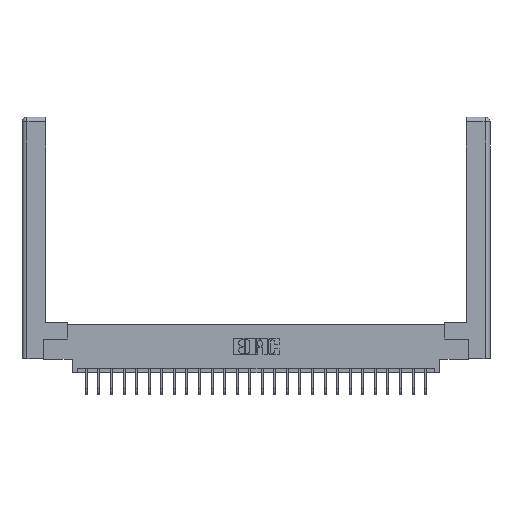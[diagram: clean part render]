
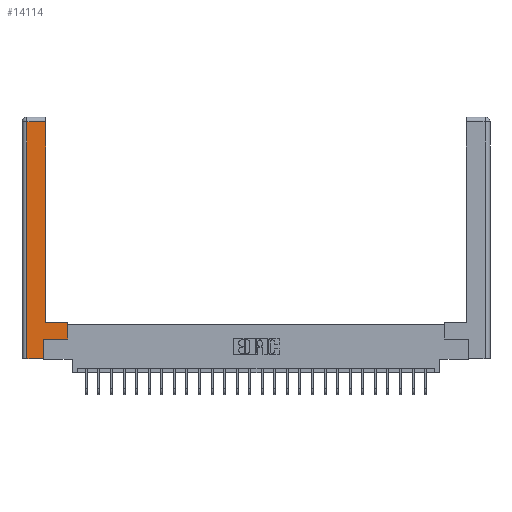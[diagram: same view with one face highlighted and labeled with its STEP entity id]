
A CAD part, top view. The second image highlights one B-rep face of the part: STEP entity #14114.
In plain terms, the highlighted planar face has unit normal (0, 0, 1).
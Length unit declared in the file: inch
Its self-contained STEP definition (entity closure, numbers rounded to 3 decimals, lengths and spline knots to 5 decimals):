
#35 = ORIENTED_EDGE ( 'NONE', *, *, #8858, .T. ) ;
#504 = EDGE_CURVE ( 'NONE', #5741, #15516, #4902, .T. ) ;
#1690 = LINE ( 'NONE', #20446, #19016 ) ;
#2625 = CARTESIAN_POINT ( 'NONE',  ( 0.565, 0.245, 0. ) ) ;
#2643 = CARTESIAN_POINT ( 'NONE',  ( 0.565, 0.45, 0. ) ) ;
#2714 = ORIENTED_EDGE ( 'NONE', *, *, #23571, .T. ) ;
#3656 = VERTEX_POINT ( 'NONE', #13217 ) ;
#4498 = ORIENTED_EDGE ( 'NONE', *, *, #504, .T. ) ;
#4645 = ORIENTED_EDGE ( 'NONE', *, *, #26272, .T. ) ;
#4902 = LINE ( 'NONE', #16597, #22898 ) ;
#5548 = DIRECTION ( 'NONE',  ( 1., 0., 0. ) ) ;
#5676 = DIRECTION ( 'NONE',  ( 0., 1., 0. ) ) ;
#5741 = VERTEX_POINT ( 'NONE', #2643 ) ;
#5812 = LINE ( 'NONE', #17185, #20409 ) ;
#6780 = CARTESIAN_POINT ( 'NONE',  ( 0.0615, 2.94, 0. ) ) ;
#6883 = VERTEX_POINT ( 'NONE', #10558 ) ;
#7050 = CARTESIAN_POINT ( 'NONE',  ( 0.265, 0.245, 0. ) ) ;
#8350 = VERTEX_POINT ( 'NONE', #18207 ) ;
#8858 = EDGE_CURVE ( 'NONE', #15516, #6883, #27271, .T. ) ;
#8948 = LINE ( 'NONE', #13601, #22228 ) ;
#9142 = ORIENTED_EDGE ( 'NONE', *, *, #23802, .T. ) ;
#9517 = CARTESIAN_POINT ( 'NONE',  ( 0.0615, 2.94, 0. ) ) ;
#10075 = DIRECTION ( 'NONE',  ( -1., 0., 0. ) ) ;
#10157 = DIRECTION ( 'NONE',  ( -1., 0., 0. ) ) ;
#10325 = CARTESIAN_POINT ( 'NONE',  ( 0.295, 3., 0. ) ) ;
#10416 = VECTOR ( 'NONE', #13216, 39.37008 ) ;
#10558 = CARTESIAN_POINT ( 'NONE',  ( 0.295, 2.94, 0. ) ) ;
#11442 = DIRECTION ( 'NONE',  ( 1., 0., 0. ) ) ;
#13006 = DIRECTION ( 'NONE',  ( 0., -1., 0. ) ) ;
#13217 = CARTESIAN_POINT ( 'NONE',  ( 0.265, 0., 0. ) ) ;
#13216 = DIRECTION ( 'NONE',  ( 0., 1., 0. ) ) ;
#13601 = CARTESIAN_POINT ( 'NONE',  ( 0.265, 0., 0. ) ) ;
#14114 = ADVANCED_FACE ( 'NONE', ( #24796 ), #27382, .F. ) ;
#14404 = DIRECTION ( 'NONE',  ( 0., 0., -1. ) ) ;
#14780 = CARTESIAN_POINT ( 'NONE',  ( 0.265, 0.245, 0. ) ) ;
#15516 = VERTEX_POINT ( 'NONE', #20172 ) ;
#16261 = ORIENTED_EDGE ( 'NONE', *, *, #25699, .T. ) ;
#16597 = CARTESIAN_POINT ( 'NONE',  ( 0.295, 0.45, 0. ) ) ;
#16770 = VECTOR ( 'NONE', #21987, 39.37008 ) ;
#17185 = CARTESIAN_POINT ( 'NONE',  ( 0.0615, 0., 0. ) ) ;
#17998 = LINE ( 'NONE', #2625, #19357 ) ;
#18051 = EDGE_CURVE ( 'NONE', #3656, #27530, #19575, .T. ) ;
#18207 = CARTESIAN_POINT ( 'NONE',  ( 0.0615, 0., 0. ) ) ;
#19016 = VECTOR ( 'NONE', #26777, 39.37008 ) ;
#19269 = VERTEX_POINT ( 'NONE', #24216 ) ;
#19357 = VECTOR ( 'NONE', #11442, 39.37008 ) ;
#19500 = LINE ( 'NONE', #6780, #16770 ) ;
#19575 = LINE ( 'NONE', #7050, #10416 ) ;
#20172 = CARTESIAN_POINT ( 'NONE',  ( 0.295, 0.45, 0. ) ) ;
#20409 = VECTOR ( 'NONE', #13006, 39.37008 ) ;
#20446 = CARTESIAN_POINT ( 'NONE',  ( 0.565, 0.45, 0. ) ) ;
#20971 = CARTESIAN_POINT ( 'NONE',  ( 0., 0., 0. ) ) ;
#21510 = VERTEX_POINT ( 'NONE', #9517 ) ;
#21685 = ORIENTED_EDGE ( 'NONE', *, *, #26154, .T. ) ;
#21987 = DIRECTION ( 'NONE',  ( -1., 0., 0. ) ) ;
#22228 = VECTOR ( 'NONE', #5548, 39.37008 ) ;
#22583 = AXIS2_PLACEMENT_3D ( 'NONE', #20971, #14404, #10157 ) ;
#22898 = VECTOR ( 'NONE', #10075, 39.37008 ) ;
#23571 = EDGE_CURVE ( 'NONE', #6883, #21510, #19500, .T. ) ;
#23802 = EDGE_CURVE ( 'NONE', #8350, #3656, #8948, .T. ) ;
#24143 = ORIENTED_EDGE ( 'NONE', *, *, #18051, .T. ) ;
#24216 = CARTESIAN_POINT ( 'NONE',  ( 0.565, 0.245, 0. ) ) ;
#24796 = FACE_OUTER_BOUND ( 'NONE', #27356, .T. ) ;
#25699 = EDGE_CURVE ( 'NONE', #21510, #8350, #5812, .T. ) ;
#25932 = VECTOR ( 'NONE', #5676, 39.37008 ) ;
#26154 = EDGE_CURVE ( 'NONE', #27530, #19269, #17998, .T. ) ;
#26272 = EDGE_CURVE ( 'NONE', #19269, #5741, #1690, .T. ) ;
#26777 = DIRECTION ( 'NONE',  ( 0., 1., 0. ) ) ;
#27271 = LINE ( 'NONE', #10325, #25932 ) ;
#27356 = EDGE_LOOP ( 'NONE', ( #35, #2714, #16261, #9142, #24143, #21685, #4645, #4498 ) ) ;
#27382 = PLANE ( 'NONE',  #22583 ) ;
#27530 = VERTEX_POINT ( 'NONE', #14780 ) ;
